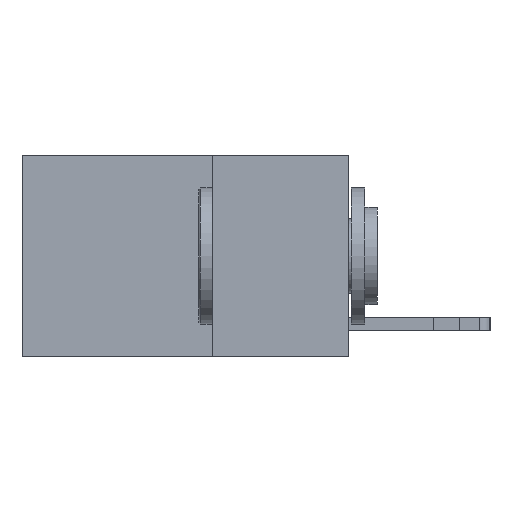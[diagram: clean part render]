
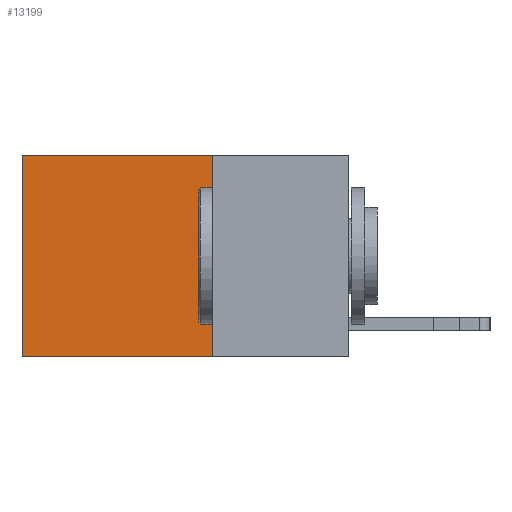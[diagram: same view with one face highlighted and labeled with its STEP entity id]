
A CAD part, left-side view. The second image highlights one B-rep face of the part: STEP entity #13199.
In plain terms, the highlighted planar face has unit normal (-1, 0, 0).
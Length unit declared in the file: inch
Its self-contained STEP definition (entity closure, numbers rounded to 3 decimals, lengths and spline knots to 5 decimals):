
#1381 = EDGE_CURVE ( 'NONE', #15455, #4366, #1760, .T. ) ;
#1388 = CARTESIAN_POINT ( 'NONE',  ( 0.2625, 0.25, 0. ) ) ;
#1412 = CARTESIAN_POINT ( 'NONE',  ( 0.2625, 0.25, -0.37 ) ) ;
#1760 = LINE ( 'NONE', #21787, #7562 ) ;
#1879 = EDGE_LOOP ( 'NONE', ( #16358, #15424, #6118, #14350 ) ) ;
#2567 = EDGE_CURVE ( 'NONE', #15848, #15455, #6136, .T. ) ;
#3086 = FACE_OUTER_BOUND ( 'NONE', #1879, .T. ) ;
#3430 = DIRECTION ( 'NONE',  ( 1., 0., 0. ) ) ;
#3541 = PLANE ( 'NONE',  #5351 ) ;
#3728 = VECTOR ( 'NONE', #14483, 39.37008 ) ;
#4366 = VERTEX_POINT ( 'NONE', #15736 ) ;
#4383 = VECTOR ( 'NONE', #11429, 39.37008 ) ;
#5015 = VERTEX_POINT ( 'NONE', #19640 ) ;
#5351 = AXIS2_PLACEMENT_3D ( 'NONE', #6662, #3430, #10638 ) ;
#6118 = ORIENTED_EDGE ( 'NONE', *, *, #2567, .F. ) ;
#6136 = LINE ( 'NONE', #20534, #4383 ) ;
#6662 = CARTESIAN_POINT ( 'NONE',  ( 0.2625, 0.25, 0. ) ) ;
#7562 = VECTOR ( 'NONE', #19994, 39.37008 ) ;
#10638 = DIRECTION ( 'NONE',  ( 0., 0., -1. ) ) ;
#10749 = LINE ( 'NONE', #14972, #3728 ) ;
#11017 = DIRECTION ( 'NONE',  ( 0., 1., 0. ) ) ;
#11429 = DIRECTION ( 'NONE',  ( 0., 0., -1. ) ) ;
#12892 = EDGE_CURVE ( 'NONE', #15848, #5015, #15016, .T. ) ;
#13199 = ADVANCED_FACE ( 'NONE', ( #3086 ), #3541, .F. ) ;
#13786 = VECTOR ( 'NONE', #11017, 39.37008 ) ;
#14350 = ORIENTED_EDGE ( 'NONE', *, *, #12892, .T. ) ;
#14483 = DIRECTION ( 'NONE',  ( 0., 0., -1. ) ) ;
#14972 = CARTESIAN_POINT ( 'NONE',  ( 0.2625, 0.6, 0. ) ) ;
#15016 = LINE ( 'NONE', #16562, #13786 ) ;
#15424 = ORIENTED_EDGE ( 'NONE', *, *, #1381, .F. ) ;
#15455 = VERTEX_POINT ( 'NONE', #1412 ) ;
#15736 = CARTESIAN_POINT ( 'NONE',  ( 0.2625, 0.6, -0.37 ) ) ;
#15848 = VERTEX_POINT ( 'NONE', #1388 ) ;
#16358 = ORIENTED_EDGE ( 'NONE', *, *, #20679, .T. ) ;
#16562 = CARTESIAN_POINT ( 'NONE',  ( 0.2625, 0.25, 0. ) ) ;
#19640 = CARTESIAN_POINT ( 'NONE',  ( 0.2625, 0.6, 0. ) ) ;
#19994 = DIRECTION ( 'NONE',  ( 0., 1., 0. ) ) ;
#20534 = CARTESIAN_POINT ( 'NONE',  ( 0.2625, 0.25, 0. ) ) ;
#20679 = EDGE_CURVE ( 'NONE', #5015, #4366, #10749, .T. ) ;
#21787 = CARTESIAN_POINT ( 'NONE',  ( 0.2625, 0.25, -0.37 ) ) ;
